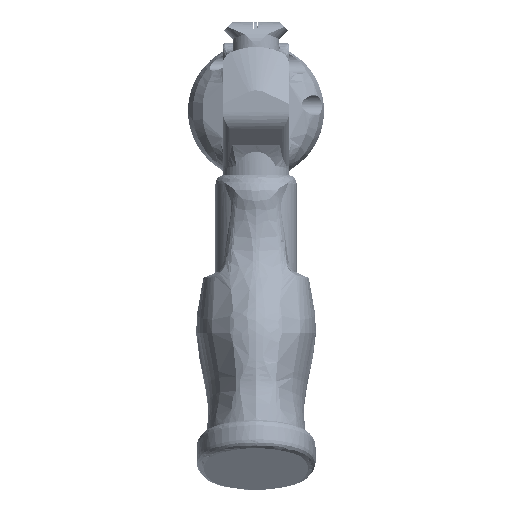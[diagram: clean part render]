
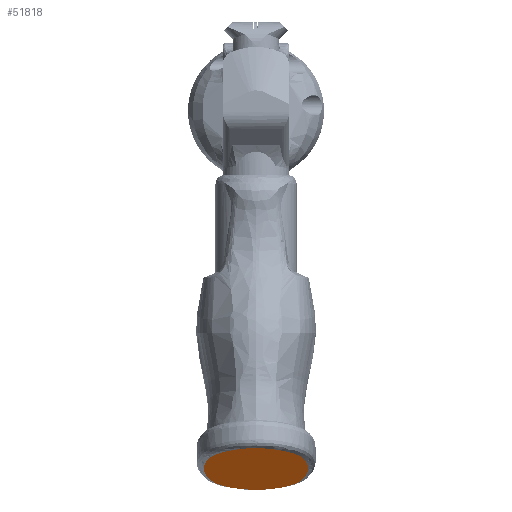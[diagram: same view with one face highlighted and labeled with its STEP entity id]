
A CAD part, left-side view. The second image highlights one B-rep face of the part: STEP entity #51818.
In plain terms, the highlighted planar face has unit normal (-0.259, 0, -0.966).
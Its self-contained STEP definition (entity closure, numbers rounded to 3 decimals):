
#3169=B_SPLINE_CURVE_WITH_KNOTS('',3,(#159317,#159318,#159319,#159320,#159321,
#159322,#159323,#159324,#159325,#159326,#159327,#159328,#159329,#159330,
#159331,#159332,#159333,#159334,#159335,#159336,#159337,#159338,#159339,
#159340,#159341,#159342,#159343,#159344,#159345,#159346,#159347,#159348,
#159349,#159350,#159351,#159352,#159353,#159354,#159355,#159356,#159357,
#159358,#159359),.UNSPECIFIED.,.F.,.F.,(4,2,2,1,1,2,2,2,2,2,1,2,2,2,2,2,
1,2,2,2,1,2,2,4),(0.006,0.019,0.572,
0.597,0.912,1.167,1.831,2.109,
2.578,3.454,3.481,3.884,4.134,
4.709,4.967,5.471,5.557,6.204,
6.731,6.892,6.95,7.028,7.341,
7.351),.UNSPECIFIED.);
#3174=B_SPLINE_CURVE_WITH_KNOTS('',3,(#160132,#160133,#160134,#160135,#160136,
#160137,#160138,#160139,#160140,#160141,#160142,#160143,#160144,#160145,
#160146,#160147,#160148,#160149,#160150,#160151,#160152,#160153,#160154,
#160155,#160156,#160157,#160158,#160159,#160160,#160161,#160162,#160163,
#160164,#160165,#160166,#160167,#160168,#160169,#160170,#160171),
 .UNSPECIFIED.,.F.,.F.,(4,2,2,2,1,2,2,1,2,2,2,1,2,2,2,1,1,2,1,2,2,2,4),
(0.005,0.015,0.356,0.55,
1.005,1.346,1.422,1.811,2.103,
2.274,2.794,3.528,4.506,5.04,
5.1,5.111,5.422,5.851,6.245,
6.541,6.928,7.33,7.342),
 .UNSPECIFIED.);
#4973=PLANE('',#56069);
#8065=FACE_OUTER_BOUND('',#11063,.T.);
#11063=EDGE_LOOP('',(#45647,#45648));
#23582=VERTEX_POINT('',#159315);
#23583=VERTEX_POINT('',#159316);
#31190=EDGE_CURVE('',#23582,#23583,#3169,.T.);
#31195=EDGE_CURVE('',#23583,#23582,#3174,.T.);
#45647=ORIENTED_EDGE('',*,*,#31190,.F.);
#45648=ORIENTED_EDGE('',*,*,#31195,.F.);
#51818=ADVANCED_FACE('',(#8065),#4973,.T.);
#56069=AXIS2_PLACEMENT_3D('',#161166,#66252,#66253);
#66252=DIRECTION('center_axis',(-0.259,0.,
-0.966));
#66253=DIRECTION('ref_axis',(0.,-1.,0.));
#159315=CARTESIAN_POINT('',(32.882,-157.25,88.674));
#159316=CARTESIAN_POINT('',(-20.756,-157.25,103.064));
#159317=CARTESIAN_POINT('Ctrl Pts',(32.882,-157.25,88.674));
#159318=CARTESIAN_POINT('Ctrl Pts',(32.881,-157.207,
88.674));
#159319=CARTESIAN_POINT('Ctrl Pts',(32.879,-157.165,
88.674));
#159320=CARTESIAN_POINT('Ctrl Pts',(32.833,-155.278,88.687));
#159321=CARTESIAN_POINT('Ctrl Pts',(32.449,-153.446,
88.79));
#159322=CARTESIAN_POINT('Ctrl Pts',(31.737,-151.651,
88.981));
#159323=CARTESIAN_POINT('Ctrl Pts',(31.309,-150.596,
89.096));
#159324=CARTESIAN_POINT('Ctrl Pts',(30.365,-148.833,89.349));
#159325=CARTESIAN_POINT('Ctrl Pts',(29.21,-147.352,89.659));
#159326=CARTESIAN_POINT('Ctrl Pts',(27.179,-145.097,
90.204));
#159327=CARTESIAN_POINT('Ctrl Pts',(25.41,-143.763,
90.678));
#159328=CARTESIAN_POINT('Ctrl Pts',(22.707,-142.346,91.403));
#159329=CARTESIAN_POINT('Ctrl Pts',(21.883,-141.976,91.625));
#159330=CARTESIAN_POINT('Ctrl Pts',(19.595,-141.157,
92.238));
#159331=CARTESIAN_POINT('Ctrl Pts',(18.104,-140.785,92.639));
#159332=CARTESIAN_POINT('Ctrl Pts',(13.816,-139.821,
93.789));
#159333=CARTESIAN_POINT('Ctrl Pts',(11.021,-139.412,94.539));
#159334=CARTESIAN_POINT('Ctrl Pts',(8.105,-139.246,
95.321));
#159335=CARTESIAN_POINT('Ctrl Pts',(6.716,-139.171,
95.694));
#159336=CARTESIAN_POINT('Ctrl Pts',(5.323,-139.156,96.068));
#159337=CARTESIAN_POINT('Ctrl Pts',(3.21,-139.215,
96.634));
#159338=CARTESIAN_POINT('Ctrl Pts',(2.405,-139.257,
96.85));
#159339=CARTESIAN_POINT('Ctrl Pts',(-0.254,-139.463,
97.564));
#159340=CARTESIAN_POINT('Ctrl Pts',(-2.091,-139.713,
98.057));
#159341=CARTESIAN_POINT('Ctrl Pts',(-4.746,-140.207,
98.769));
#159342=CARTESIAN_POINT('Ctrl Pts',(-5.561,-140.39,
98.988));
#159343=CARTESIAN_POINT('Ctrl Pts',(-7.944,-141.033,
99.627));
#159344=CARTESIAN_POINT('Ctrl Pts',(-9.486,-141.578,
100.041));
#159345=CARTESIAN_POINT('Ctrl Pts',(-11.184,-142.482,
100.496));
#159346=CARTESIAN_POINT('Ctrl Pts',(-13.267,-143.655,
101.055));
#159347=CARTESIAN_POINT('Ctrl Pts',(-15.122,-145.243,
101.553));
#159348=CARTESIAN_POINT('Ctrl Pts',(-17.614,-148.204,
102.221));
#159349=CARTESIAN_POINT('Ctrl Pts',(-18.556,-149.682,
102.474));
#159350=CARTESIAN_POINT('Ctrl Pts',(-19.536,-151.753,
102.737));
#159351=CARTESIAN_POINT('Ctrl Pts',(-19.748,-152.249,
102.794));
#159352=CARTESIAN_POINT('Ctrl Pts',(-19.999,-152.936,
102.861));
#159353=CARTESIAN_POINT('Ctrl Pts',(-20.144,-153.362,
102.9));
#159354=CARTESIAN_POINT('Ctrl Pts',(-20.271,-153.794,
102.934));
#159355=CARTESIAN_POINT('Ctrl Pts',(-20.592,-155.054,
103.02));
#159356=CARTESIAN_POINT('Ctrl Pts',(-20.733,-156.102,
103.058));
#159357=CARTESIAN_POINT('Ctrl Pts',(-20.755,-157.181,
103.064));
#159358=CARTESIAN_POINT('Ctrl Pts',(-20.755,-157.216,
103.064));
#159359=CARTESIAN_POINT('Ctrl Pts',(-20.756,-157.25,
103.064));
#160132=CARTESIAN_POINT('Ctrl Pts',(-20.756,-157.25,
103.064));
#160133=CARTESIAN_POINT('Ctrl Pts',(-20.755,-157.284,
103.064));
#160134=CARTESIAN_POINT('Ctrl Pts',(-20.755,-157.319,
103.064));
#160135=CARTESIAN_POINT('Ctrl Pts',(-20.731,-158.488,
103.058));
#160136=CARTESIAN_POINT('Ctrl Pts',(-20.566,-159.63,
103.013));
#160137=CARTESIAN_POINT('Ctrl Pts',(-20.09,-161.346,
102.886));
#160138=CARTESIAN_POINT('Ctrl Pts',(-19.87,-161.954,
102.827));
#160139=CARTESIAN_POINT('Ctrl Pts',(-19.017,-163.94,
102.598));
#160140=CARTESIAN_POINT('Ctrl Pts',(-17.697,-166.275,
102.244));
#160141=CARTESIAN_POINT('Ctrl Pts',(-15.982,-168.259,
101.784));
#160142=CARTESIAN_POINT('Ctrl Pts',(-14.995,-169.22,
101.519));
#160143=CARTESIAN_POINT('Ctrl Pts',(-14.812,-169.392,
101.47));
#160144=CARTESIAN_POINT('Ctrl Pts',(-13.674,-170.421,
101.164));
#160145=CARTESIAN_POINT('Ctrl Pts',(-11.848,-171.746,
100.674));
#160146=CARTESIAN_POINT('Ctrl Pts',(-9.863,-172.705,
100.142));
#160147=CARTESIAN_POINT('Ctrl Pts',(-8.467,-173.245,
99.767));
#160148=CARTESIAN_POINT('Ctrl Pts',(-7.946,-173.428,
99.627));
#160149=CARTESIAN_POINT('Ctrl Pts',(-5.808,-174.093,
99.054));
#160150=CARTESIAN_POINT('Ctrl Pts',(-4.141,-174.431,
98.606));
#160151=CARTESIAN_POINT('Ctrl Pts',(-0.107,-175.073,
97.524));
#160152=CARTESIAN_POINT('Ctrl Pts',(5.389,-175.566,
96.05));
#160153=CARTESIAN_POINT('Ctrl Pts',(10.963,-175.11,
94.554));
#160154=CARTESIAN_POINT('Ctrl Pts',(15.784,-174.258,
93.261));
#160155=CARTESIAN_POINT('Ctrl Pts',(17.458,-173.877,
92.812));
#160156=CARTESIAN_POINT('Ctrl Pts',(19.327,-173.376,
92.31));
#160157=CARTESIAN_POINT('Ctrl Pts',(19.515,-173.323,92.26));
#160158=CARTESIAN_POINT('Ctrl Pts',(19.737,-173.257,
92.2));
#160159=CARTESIAN_POINT('Ctrl Pts',(20.746,-172.957,91.93));
#160160=CARTESIAN_POINT('Ctrl Pts',(23.057,-172.074,
91.31));
#160161=CARTESIAN_POINT('Ctrl Pts',(25.138,-170.838,
90.751));
#160162=CARTESIAN_POINT('Ctrl Pts',(27.271,-169.202,
90.179));
#160163=CARTESIAN_POINT('Ctrl Pts',(28.932,-167.617,
89.733));
#160164=CARTESIAN_POINT('Ctrl Pts',(30.246,-165.752,
89.381));
#160165=CARTESIAN_POINT('Ctrl Pts',(31.379,-163.788,
89.077));
#160166=CARTESIAN_POINT('Ctrl Pts',(31.897,-162.583,88.938));
#160167=CARTESIAN_POINT('Ctrl Pts',(32.635,-160.048,
88.74));
#160168=CARTESIAN_POINT('Ctrl Pts',(32.845,-158.717,
88.683));
#160169=CARTESIAN_POINT('Ctrl Pts',(32.879,-157.335,
88.674));
#160170=CARTESIAN_POINT('Ctrl Pts',(32.881,-157.293,
88.674));
#160171=CARTESIAN_POINT('Ctrl Pts',(32.882,-157.25,
88.674));
#161166=CARTESIAN_POINT('Origin',(6.063,-157.388,95.869));
